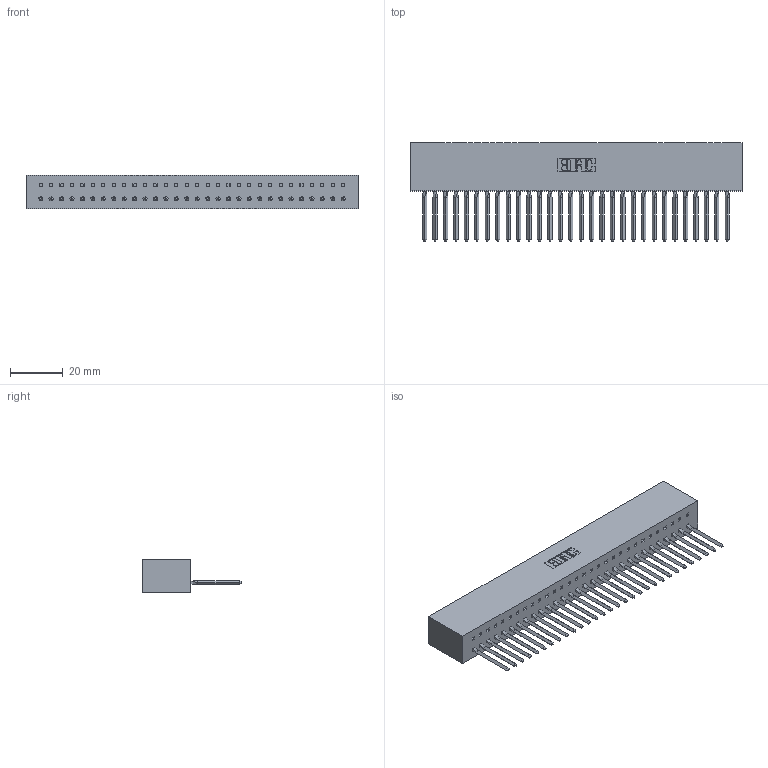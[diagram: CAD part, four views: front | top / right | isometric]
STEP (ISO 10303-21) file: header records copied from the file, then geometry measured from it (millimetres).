
FILE_DESCRIPTION (( 'STEP AP203' ), '1' );
FILE_NAME ('317-030-541-601.STEP', '2020-02-27T20:11:11', ( '' ), ( '' ), 'SwSTEP 2.0', 'SolidWorks 2016', '' );
FILE_SCHEMA (( 'CONFIG_CONTROL_DESIGN' ));
Length unit declared in the file: inch
Products named in the file (3): 317-290-002_541; 317 Part_Lugless; 317-030-541-601
Assembly tree (31 placements, depth 2):
  317-030-541-601
    317 Part_Lugless
    317-290-002_541  x30
Bounding box: 126.09 x 37.34 x 12.7 mm (x, y, z)
Volume: 21783.7 mm3; surface area: 30575.4 mm2
Topology: 31 solids, 31 shells, 4650 faces, 13259 edges, 8618 vertices
Faces by surface type: plane 3770, cylinder 760, bspline 120
Entity records: 45218 total; most frequent: CARTESIAN_POINT 8675, ORIENTED_EDGE 7958, DIRECTION 6519, EDGE_CURVE 3979, VECTOR 3623, LINE 3623, VERTEX_POINT 2644, AXIS2_PLACEMENT_3D 1448
